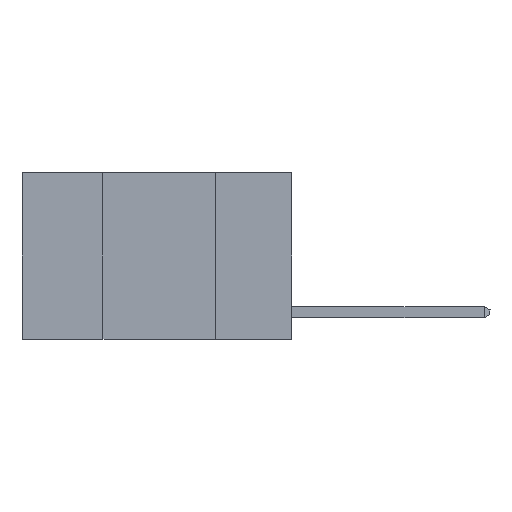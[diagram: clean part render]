
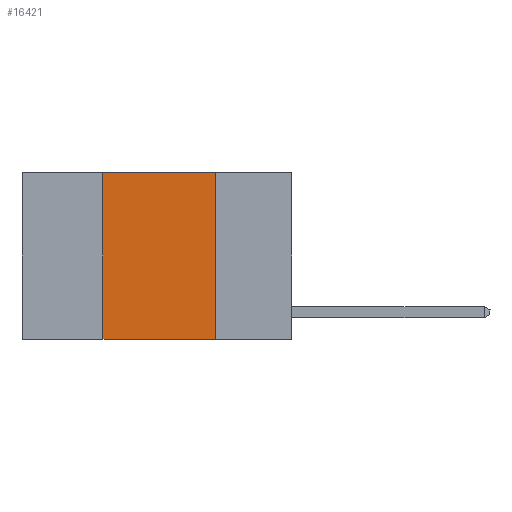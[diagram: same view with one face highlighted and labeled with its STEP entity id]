
A CAD part, left-side view. The second image highlights one B-rep face of the part: STEP entity #16421.
In plain terms, the highlighted planar face has unit normal (-1, 0, 0).
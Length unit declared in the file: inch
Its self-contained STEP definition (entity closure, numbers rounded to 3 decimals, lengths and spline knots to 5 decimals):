
#371 = VECTOR ( 'NONE', #2248, 39.37008 ) ;
#375 = CARTESIAN_POINT ( 'NONE',  ( 0., 0.17, 0. ) ) ;
#2115 = EDGE_CURVE ( 'NONE', #4545, #6781, #16569, .T. ) ;
#2248 = DIRECTION ( 'NONE',  ( 0., -1., 0. ) ) ;
#2920 = ORIENTED_EDGE ( 'NONE', *, *, #11098, .F. ) ;
#3101 = FACE_OUTER_BOUND ( 'NONE', #15968, .T. ) ;
#3639 = CARTESIAN_POINT ( 'NONE',  ( 0., 0.17, -0.37 ) ) ;
#4395 = DIRECTION ( 'NONE',  ( 0., 0., 1. ) ) ;
#4522 = CARTESIAN_POINT ( 'NONE',  ( 0., 0.42, -0.37 ) ) ;
#4545 = VERTEX_POINT ( 'NONE', #4522 ) ;
#4809 = CARTESIAN_POINT ( 'NONE',  ( 0., 0.42, 0. ) ) ;
#4981 = LINE ( 'NONE', #10359, #371 ) ;
#5649 = EDGE_CURVE ( 'NONE', #15790, #7852, #11521, .T. ) ;
#5731 = VECTOR ( 'NONE', #16629, 39.37008 ) ;
#5904 = VECTOR ( 'NONE', #4395, 39.37008 ) ;
#6587 = CARTESIAN_POINT ( 'NONE',  ( 0., 0.6, -0.37 ) ) ;
#6781 = VERTEX_POINT ( 'NONE', #4809 ) ;
#7340 = CARTESIAN_POINT ( 'NONE',  ( 0., 0.6, 0. ) ) ;
#7822 = LINE ( 'NONE', #6587, #12347 ) ;
#7852 = VERTEX_POINT ( 'NONE', #3639 ) ;
#8288 = CARTESIAN_POINT ( 'NONE',  ( 0., 0.42, 0. ) ) ;
#8637 = PLANE ( 'NONE',  #10084 ) ;
#10084 = AXIS2_PLACEMENT_3D ( 'NONE', #7340, #15437, #14019 ) ;
#10320 = ORIENTED_EDGE ( 'NONE', *, *, #2115, .F. ) ;
#10359 = CARTESIAN_POINT ( 'NONE',  ( 0., 0.6, 0. ) ) ;
#10638 = ORIENTED_EDGE ( 'NONE', *, *, #17084, .T. ) ;
#11098 = EDGE_CURVE ( 'NONE', #6781, #15790, #4981, .T. ) ;
#11337 = CARTESIAN_POINT ( 'NONE',  ( 0., 0.17, 0. ) ) ;
#11521 = LINE ( 'NONE', #11337, #5731 ) ;
#12347 = VECTOR ( 'NONE', #13193, 39.37008 ) ;
#13193 = DIRECTION ( 'NONE',  ( 0., -1., 0. ) ) ;
#14019 = DIRECTION ( 'NONE',  ( 0., 0., -1. ) ) ;
#15437 = DIRECTION ( 'NONE',  ( 1., 0., 0. ) ) ;
#15727 = ORIENTED_EDGE ( 'NONE', *, *, #5649, .F. ) ;
#15790 = VERTEX_POINT ( 'NONE', #375 ) ;
#15968 = EDGE_LOOP ( 'NONE', ( #15727, #2920, #10320, #10638 ) ) ;
#16421 = ADVANCED_FACE ( 'NONE', ( #3101 ), #8637, .F. ) ;
#16569 = LINE ( 'NONE', #8288, #5904 ) ;
#16629 = DIRECTION ( 'NONE',  ( 0., 0., -1. ) ) ;
#17084 = EDGE_CURVE ( 'NONE', #4545, #7852, #7822, .T. ) ;
